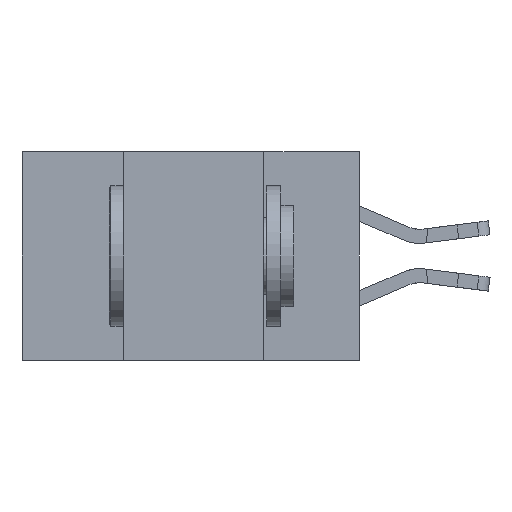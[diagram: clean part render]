
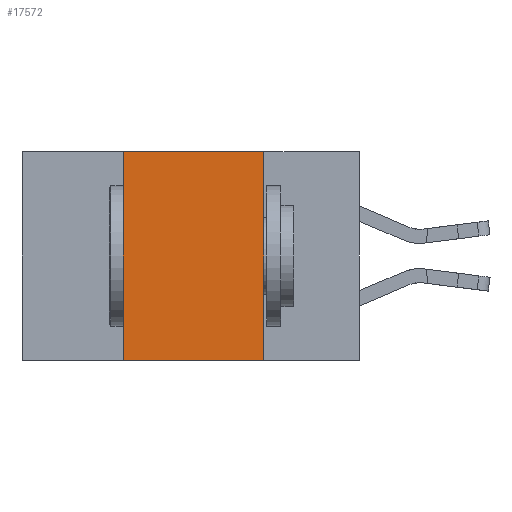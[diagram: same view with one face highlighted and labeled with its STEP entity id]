
A CAD part, left-side view. The second image highlights one B-rep face of the part: STEP entity #17572.
In plain terms, the highlighted planar face has unit normal (-1, 0, 0).
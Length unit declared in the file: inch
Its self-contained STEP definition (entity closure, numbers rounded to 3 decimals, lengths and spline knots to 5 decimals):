
#1321 = DIRECTION ( 'NONE',  ( 0., -1., 0. ) ) ;
#1428 = CARTESIAN_POINT ( 'NONE',  ( 0., 0.17, 0. ) ) ;
#1509 = CARTESIAN_POINT ( 'NONE',  ( 0., 0.42, 0. ) ) ;
#3044 = DIRECTION ( 'NONE',  ( 1., 0., 0. ) ) ;
#4036 = EDGE_CURVE ( 'NONE', #16467, #8571, #12725, .T. ) ;
#4227 = CARTESIAN_POINT ( 'NONE',  ( 0., 0.6, -0.37 ) ) ;
#4229 = ORIENTED_EDGE ( 'NONE', *, *, #21285, .F. ) ;
#5227 = VECTOR ( 'NONE', #13048, 39.37008 ) ;
#5750 = LINE ( 'NONE', #19628, #5227 ) ;
#6022 = AXIS2_PLACEMENT_3D ( 'NONE', #6476, #3044, #19813 ) ;
#6476 = CARTESIAN_POINT ( 'NONE',  ( 0., 0.6, 0. ) ) ;
#6737 = VECTOR ( 'NONE', #19903, 39.37008 ) ;
#7660 = DIRECTION ( 'NONE',  ( 0., -1., 0. ) ) ;
#8109 = CARTESIAN_POINT ( 'NONE',  ( 0., 0.6, 0. ) ) ;
#8172 = PLANE ( 'NONE',  #6022 ) ;
#8280 = VECTOR ( 'NONE', #1321, 39.37008 ) ;
#8571 = VERTEX_POINT ( 'NONE', #9651 ) ;
#9651 = CARTESIAN_POINT ( 'NONE',  ( 0., 0.17, 0. ) ) ;
#9996 = ORIENTED_EDGE ( 'NONE', *, *, #4036, .F. ) ;
#10081 = EDGE_CURVE ( 'NONE', #8571, #18917, #11218, .T. ) ;
#11218 = LINE ( 'NONE', #1428, #6737 ) ;
#11424 = CARTESIAN_POINT ( 'NONE',  ( 0., 0.42, -0.37 ) ) ;
#12725 = LINE ( 'NONE', #8109, #8280 ) ;
#13048 = DIRECTION ( 'NONE',  ( 0., 0., 1. ) ) ;
#13092 = LINE ( 'NONE', #4227, #17503 ) ;
#14284 = FACE_OUTER_BOUND ( 'NONE', #14760, .T. ) ;
#14538 = ORIENTED_EDGE ( 'NONE', *, *, #15611, .T. ) ;
#14760 = EDGE_LOOP ( 'NONE', ( #17113, #9996, #4229, #14538 ) ) ;
#14988 = CARTESIAN_POINT ( 'NONE',  ( 0., 0.17, -0.37 ) ) ;
#15611 = EDGE_CURVE ( 'NONE', #19439, #18917, #13092, .T. ) ;
#16467 = VERTEX_POINT ( 'NONE', #1509 ) ;
#17113 = ORIENTED_EDGE ( 'NONE', *, *, #10081, .F. ) ;
#17503 = VECTOR ( 'NONE', #7660, 39.37008 ) ;
#17572 = ADVANCED_FACE ( 'NONE', ( #14284 ), #8172, .F. ) ;
#18917 = VERTEX_POINT ( 'NONE', #14988 ) ;
#19439 = VERTEX_POINT ( 'NONE', #11424 ) ;
#19628 = CARTESIAN_POINT ( 'NONE',  ( 0., 0.42, 0. ) ) ;
#19813 = DIRECTION ( 'NONE',  ( 0., 0., -1. ) ) ;
#19903 = DIRECTION ( 'NONE',  ( 0., 0., -1. ) ) ;
#21285 = EDGE_CURVE ( 'NONE', #19439, #16467, #5750, .T. ) ;
